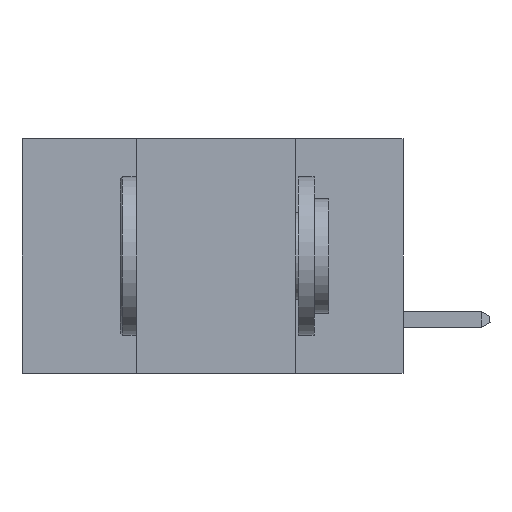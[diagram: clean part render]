
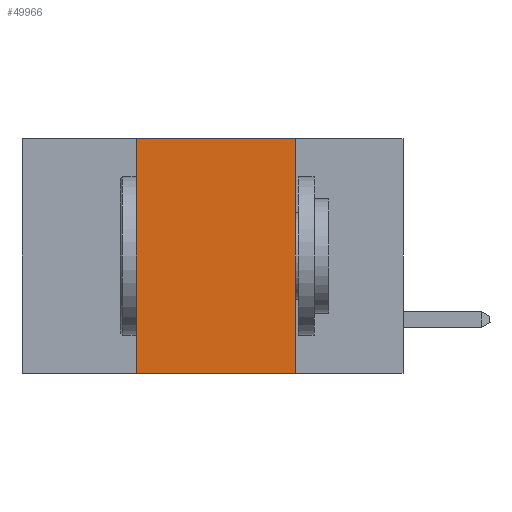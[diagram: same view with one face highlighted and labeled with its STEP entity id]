
A CAD part, left-side view. The second image highlights one B-rep face of the part: STEP entity #49966.
In plain terms, the highlighted planar face has unit normal (-1, 0, 0).
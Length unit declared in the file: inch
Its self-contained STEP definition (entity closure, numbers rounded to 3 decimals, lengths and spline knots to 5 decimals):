
#4898 = DIRECTION ( 'NONE',  ( 0., -1., 0. ) ) ;
#5070 = DIRECTION ( 'NONE',  ( 0., -1., 0. ) ) ;
#5875 = DIRECTION ( 'NONE',  ( 0., 0., -1. ) ) ;
#9933 = ORIENTED_EDGE ( 'NONE', *, *, #33170, .F. ) ;
#10665 = DIRECTION ( 'NONE',  ( 0., 0., -1. ) ) ;
#12683 = LINE ( 'NONE', #27740, #31805 ) ;
#13138 = CARTESIAN_POINT ( 'NONE',  ( 0., 0.6, -0.37 ) ) ;
#15522 = VERTEX_POINT ( 'NONE', #42778 ) ;
#15618 = ORIENTED_EDGE ( 'NONE', *, *, #35020, .T. ) ;
#16077 = VERTEX_POINT ( 'NONE', #20539 ) ;
#17416 = CARTESIAN_POINT ( 'NONE',  ( 0., 0.6, 0. ) ) ;
#18178 = LINE ( 'NONE', #40741, #26805 ) ;
#18919 = LINE ( 'NONE', #37128, #42271 ) ;
#20130 = VERTEX_POINT ( 'NONE', #50656 ) ;
#20539 = CARTESIAN_POINT ( 'NONE',  ( 0., 0.17, 0. ) ) ;
#20867 = EDGE_CURVE ( 'NONE', #15522, #24971, #12683, .T. ) ;
#24971 = VERTEX_POINT ( 'NONE', #43204 ) ;
#25956 = ORIENTED_EDGE ( 'NONE', *, *, #20867, .F. ) ;
#26805 = VECTOR ( 'NONE', #5070, 39.37008 ) ;
#27740 = CARTESIAN_POINT ( 'NONE',  ( 0., 0.42, 0. ) ) ;
#28997 = AXIS2_PLACEMENT_3D ( 'NONE', #17416, #45586, #5875 ) ;
#29722 = EDGE_LOOP ( 'NONE', ( #9933, #47117, #25956, #15618 ) ) ;
#31805 = VECTOR ( 'NONE', #48108, 39.37008 ) ;
#31952 = LINE ( 'NONE', #13138, #34978 ) ;
#33170 = EDGE_CURVE ( 'NONE', #16077, #20130, #18919, .T. ) ;
#34978 = VECTOR ( 'NONE', #4898, 39.37008 ) ;
#35020 = EDGE_CURVE ( 'NONE', #15522, #20130, #31952, .T. ) ;
#36307 = FACE_OUTER_BOUND ( 'NONE', #29722, .T. ) ;
#37128 = CARTESIAN_POINT ( 'NONE',  ( 0., 0.17, 0. ) ) ;
#40741 = CARTESIAN_POINT ( 'NONE',  ( 0., 0.6, 0. ) ) ;
#41689 = EDGE_CURVE ( 'NONE', #24971, #16077, #18178, .T. ) ;
#42271 = VECTOR ( 'NONE', #10665, 39.37008 ) ;
#42778 = CARTESIAN_POINT ( 'NONE',  ( 0., 0.42, -0.37 ) ) ;
#43204 = CARTESIAN_POINT ( 'NONE',  ( 0., 0.42, 0. ) ) ;
#45395 = PLANE ( 'NONE',  #28997 ) ;
#45586 = DIRECTION ( 'NONE',  ( 1., 0., 0. ) ) ;
#47117 = ORIENTED_EDGE ( 'NONE', *, *, #41689, .F. ) ;
#48108 = DIRECTION ( 'NONE',  ( 0., 0., 1. ) ) ;
#49966 = ADVANCED_FACE ( 'NONE', ( #36307 ), #45395, .F. ) ;
#50656 = CARTESIAN_POINT ( 'NONE',  ( 0., 0.17, -0.37 ) ) ;
